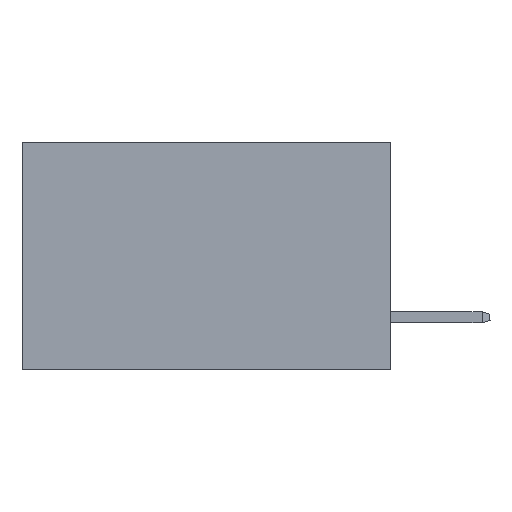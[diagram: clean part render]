
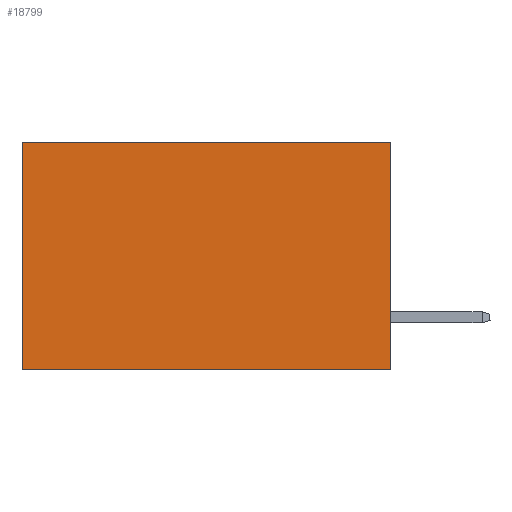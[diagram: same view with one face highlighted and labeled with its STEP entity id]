
A CAD part, left-side view. The second image highlights one B-rep face of the part: STEP entity #18799.
In plain terms, the highlighted planar face has unit normal (-1, 0, 0).
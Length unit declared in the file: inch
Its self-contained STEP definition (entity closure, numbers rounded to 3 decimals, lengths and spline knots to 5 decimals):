
#165 = CARTESIAN_POINT ( 'NONE',  ( 0.2875, 0., 0. ) ) ;
#597 = VECTOR ( 'NONE', #2486, 39.37008 ) ;
#1247 = CARTESIAN_POINT ( 'NONE',  ( 0.2875, 0., 0. ) ) ;
#1343 = CARTESIAN_POINT ( 'NONE',  ( 0.2875, 0., -0.37 ) ) ;
#1570 = LINE ( 'NONE', #11678, #12786 ) ;
#2486 = DIRECTION ( 'NONE',  ( 0., 1., 0. ) ) ;
#2600 = ORIENTED_EDGE ( 'NONE', *, *, #16288, .T. ) ;
#4224 = CARTESIAN_POINT ( 'NONE',  ( 0.2875, 0.6, -0.37 ) ) ;
#5237 = FACE_OUTER_BOUND ( 'NONE', #7292, .T. ) ;
#7292 = EDGE_LOOP ( 'NONE', ( #23664, #14156, #21596, #2600 ) ) ;
#7626 = VERTEX_POINT ( 'NONE', #17645 ) ;
#10339 = DIRECTION ( 'NONE',  ( 0., 0., -1. ) ) ;
#11678 = CARTESIAN_POINT ( 'NONE',  ( 0.2875, 0.6, 0. ) ) ;
#12786 = VECTOR ( 'NONE', #27242, 39.37008 ) ;
#13636 = VECTOR ( 'NONE', #23720, 39.37008 ) ;
#14156 = ORIENTED_EDGE ( 'NONE', *, *, #26383, .F. ) ;
#15981 = EDGE_CURVE ( 'NONE', #18237, #16623, #19572, .T. ) ;
#16288 = EDGE_CURVE ( 'NONE', #18237, #7626, #23651, .T. ) ;
#16623 = VERTEX_POINT ( 'NONE', #1343 ) ;
#16785 = VERTEX_POINT ( 'NONE', #4224 ) ;
#17335 = DIRECTION ( 'NONE',  ( 0., 1., 0. ) ) ;
#17645 = CARTESIAN_POINT ( 'NONE',  ( 0.2875, 0.6, 0. ) ) ;
#18237 = VERTEX_POINT ( 'NONE', #1247 ) ;
#18799 = ADVANCED_FACE ( 'NONE', ( #5237 ), #21104, .F. ) ;
#19315 = CARTESIAN_POINT ( 'NONE',  ( 0.2875, 0., 0. ) ) ;
#19572 = LINE ( 'NONE', #19315, #13636 ) ;
#21104 = PLANE ( 'NONE',  #22354 ) ;
#21596 = ORIENTED_EDGE ( 'NONE', *, *, #15981, .F. ) ;
#21979 = VECTOR ( 'NONE', #17335, 39.37008 ) ;
#22354 = AXIS2_PLACEMENT_3D ( 'NONE', #27662, #23680, #10339 ) ;
#23651 = LINE ( 'NONE', #165, #597 ) ;
#23664 = ORIENTED_EDGE ( 'NONE', *, *, #28438, .T. ) ;
#23680 = DIRECTION ( 'NONE',  ( 1., 0., 0. ) ) ;
#23720 = DIRECTION ( 'NONE',  ( 0., 0., -1. ) ) ;
#26383 = EDGE_CURVE ( 'NONE', #16623, #16785, #27853, .T. ) ;
#27242 = DIRECTION ( 'NONE',  ( 0., 0., -1. ) ) ;
#27662 = CARTESIAN_POINT ( 'NONE',  ( 0.2875, 0., 0. ) ) ;
#27853 = LINE ( 'NONE', #28376, #21979 ) ;
#28376 = CARTESIAN_POINT ( 'NONE',  ( 0.2875, 0., -0.37 ) ) ;
#28438 = EDGE_CURVE ( 'NONE', #7626, #16785, #1570, .T. ) ;
